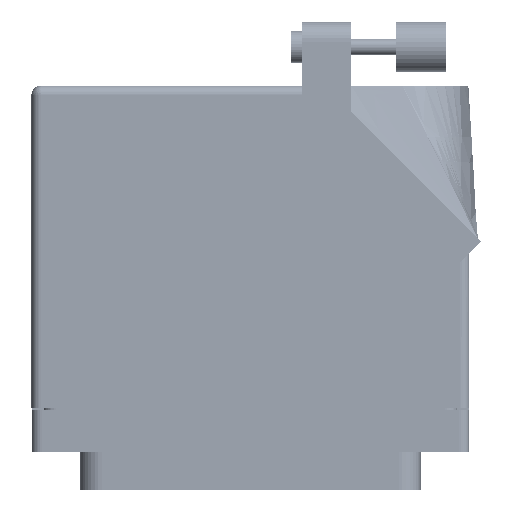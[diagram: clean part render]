
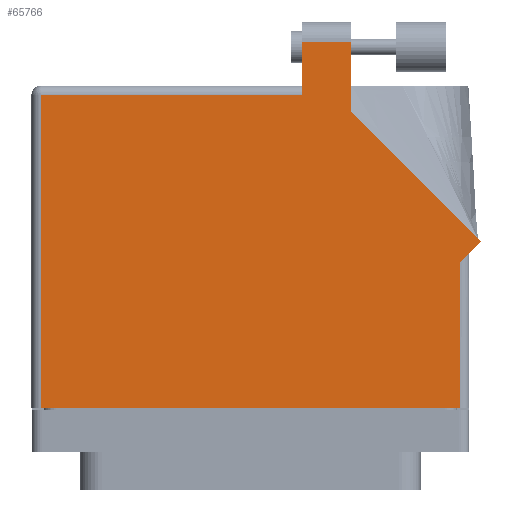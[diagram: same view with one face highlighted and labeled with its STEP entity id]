
A CAD part, front view. The second image highlights one B-rep face of the part: STEP entity #65766.
In plain terms, the highlighted face is planar.
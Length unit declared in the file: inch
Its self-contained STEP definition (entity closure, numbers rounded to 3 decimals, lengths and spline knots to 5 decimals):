
#3378 = LINE ( 'NONE', #13563, #48289 ) ;
#4003 = ORIENTED_EDGE ( 'NONE', *, *, #56324, .T. ) ;
#5532 = EDGE_CURVE ( 'NONE', #64256, #68716, #12042, .T. ) ;
#6451 = AXIS2_PLACEMENT_3D ( 'NONE', #23384, #88270, #59767 ) ;
#8261 = CARTESIAN_POINT ( 'NONE',  ( 1.3155, 0.88, 0.765 ) ) ;
#8883 = EDGE_CURVE ( 'NONE', #15031, #31165, #55671, .T. ) ;
#10979 = CARTESIAN_POINT ( 'NONE',  ( 0.6345, 2.205, 0.765 ) ) ;
#11280 = EDGE_CURVE ( 'NONE', #31165, #64256, #62016, .T. ) ;
#11384 = CARTESIAN_POINT ( 'NONE',  ( 1.3775, 0.88, 0.765 ) ) ;
#12042 = LINE ( 'NONE', #54560, #39040 ) ;
#13563 = CARTESIAN_POINT ( 'NONE',  ( -1.3775, 1.868, 0.765 ) ) ;
#13825 = ORIENTED_EDGE ( 'NONE', *, *, #61331, .T. ) ;
#14641 = ORIENTED_EDGE ( 'NONE', *, *, #55761, .T. ) ;
#15031 = VERTEX_POINT ( 'NONE', #24533 ) ;
#17042 = CARTESIAN_POINT ( 'NONE',  ( 0.3275, 2.205, 0.765 ) ) ;
#18923 = VECTOR ( 'NONE', #32976, 39.37008 ) ;
#21612 = VERTEX_POINT ( 'NONE', #10979 ) ;
#22735 = DIRECTION ( 'NONE',  ( 0., 1., 0. ) ) ;
#22743 = VECTOR ( 'NONE', #40600, 39.37008 ) ;
#23384 = CARTESIAN_POINT ( 'NONE',  ( -1.3775, 1.93, 0.765 ) ) ;
#24533 = CARTESIAN_POINT ( 'NONE',  ( 1.3155, -0.1, 0.765 ) ) ;
#24807 = CARTESIAN_POINT ( 'NONE',  ( 0.6345, 1.76442, 0.765 ) ) ;
#25360 = LINE ( 'NONE', #36308, #27630 ) ;
#27630 = VECTOR ( 'NONE', #92744, 39.37008 ) ;
#27735 = EDGE_CURVE ( 'NONE', #78099, #60787, #3378, .T. ) ;
#27756 = DIRECTION ( 'NONE',  ( -1., 0., 0. ) ) ;
#31165 = VERTEX_POINT ( 'NONE', #90264 ) ;
#31710 = VERTEX_POINT ( 'NONE', #74697 ) ;
#32976 = DIRECTION ( 'NONE',  ( 0., 1., 0. ) ) ;
#33237 = DIRECTION ( 'NONE',  ( -1., 0., 0. ) ) ;
#36308 = CARTESIAN_POINT ( 'NONE',  ( 0.3275, 1.93, 0.765 ) ) ;
#37868 = EDGE_CURVE ( 'NONE', #68716, #21612, #67226, .T. ) ;
#38247 = VERTEX_POINT ( 'NONE', #17042 ) ;
#39040 = VECTOR ( 'NONE', #82696, 39.37008 ) ;
#39179 = CARTESIAN_POINT ( 'NONE',  ( 0.3275, 1.868, 0.765 ) ) ;
#40600 = DIRECTION ( 'NONE',  ( 0.707, 0.707, 0. ) ) ;
#43627 = VECTOR ( 'NONE', #33237, 39.37008 ) ;
#43646 = ORIENTED_EDGE ( 'NONE', *, *, #37868, .T. ) ;
#43661 = EDGE_CURVE ( 'NONE', #31710, #15031, #46556, .T. ) ;
#45355 = PLANE ( 'NONE',  #6451 ) ;
#46364 = DIRECTION ( 'NONE',  ( 0., -1., 0. ) ) ;
#46556 = LINE ( 'NONE', #84373, #88033 ) ;
#48289 = VECTOR ( 'NONE', #27756, 39.37008 ) ;
#49038 = ORIENTED_EDGE ( 'NONE', *, *, #43661, .T. ) ;
#50711 = ORIENTED_EDGE ( 'NONE', *, *, #5532, .T. ) ;
#51716 = EDGE_LOOP ( 'NONE', ( #43646, #13825, #4003, #65068, #14641, #49038, #65535, #83355, #50711 ) ) ;
#54560 = CARTESIAN_POINT ( 'NONE',  ( 1.44821, 0.95071, 0.765 ) ) ;
#55671 = LINE ( 'NONE', #8261, #72469 ) ;
#55761 = EDGE_CURVE ( 'NONE', #60787, #31710, #59165, .T. ) ;
#56324 = EDGE_CURVE ( 'NONE', #38247, #78099, #25360, .T. ) ;
#59165 = LINE ( 'NONE', #81726, #76020 ) ;
#59767 = DIRECTION ( 'NONE',  ( -1., 0., 0. ) ) ;
#60787 = VERTEX_POINT ( 'NONE', #86941 ) ;
#61331 = EDGE_CURVE ( 'NONE', #21612, #38247, #82860, .T. ) ;
#62016 = LINE ( 'NONE', #11384, #22743 ) ;
#64256 = VERTEX_POINT ( 'NONE', #85707 ) ;
#65068 = ORIENTED_EDGE ( 'NONE', *, *, #27735, .T. ) ;
#65535 = ORIENTED_EDGE ( 'NONE', *, *, #8883, .T. ) ;
#65766 = ADVANCED_FACE ( 'NONE', ( #92132 ), #45355, .F. ) ;
#66848 = CARTESIAN_POINT ( 'NONE',  ( 0.6345, 1.76442, 0.765 ) ) ;
#67226 = LINE ( 'NONE', #24807, #18923 ) ;
#68716 = VERTEX_POINT ( 'NONE', #66848 ) ;
#72469 = VECTOR ( 'NONE', #22735, 39.37008 ) ;
#74697 = CARTESIAN_POINT ( 'NONE',  ( -1.3155, -0.1, 0.765 ) ) ;
#76020 = VECTOR ( 'NONE', #46364, 39.37008 ) ;
#77417 = CARTESIAN_POINT ( 'NONE',  ( 0.3275, 2.205, 0.765 ) ) ;
#78099 = VERTEX_POINT ( 'NONE', #39179 ) ;
#81726 = CARTESIAN_POINT ( 'NONE',  ( -1.3155, -0.1, 0.765 ) ) ;
#82696 = DIRECTION ( 'NONE',  ( -0.707, 0.707, 0. ) ) ;
#82860 = LINE ( 'NONE', #77417, #43627 ) ;
#83355 = ORIENTED_EDGE ( 'NONE', *, *, #11280, .T. ) ;
#84373 = CARTESIAN_POINT ( 'NONE',  ( -1.3775, -0.1, 0.765 ) ) ;
#85707 = CARTESIAN_POINT ( 'NONE',  ( 1.44821, 0.95071, 0.765 ) ) ;
#86941 = CARTESIAN_POINT ( 'NONE',  ( -1.3155, 1.868, 0.765 ) ) ;
#88033 = VECTOR ( 'NONE', #92804, 39.37008 ) ;
#88270 = DIRECTION ( 'NONE',  ( 0., 0., -1. ) ) ;
#90264 = CARTESIAN_POINT ( 'NONE',  ( 1.3155, 0.818, 0.765 ) ) ;
#92132 = FACE_OUTER_BOUND ( 'NONE', #51716, .T. ) ;
#92744 = DIRECTION ( 'NONE',  ( 0., -1., 0. ) ) ;
#92804 = DIRECTION ( 'NONE',  ( 1., 0., 0. ) ) ;
